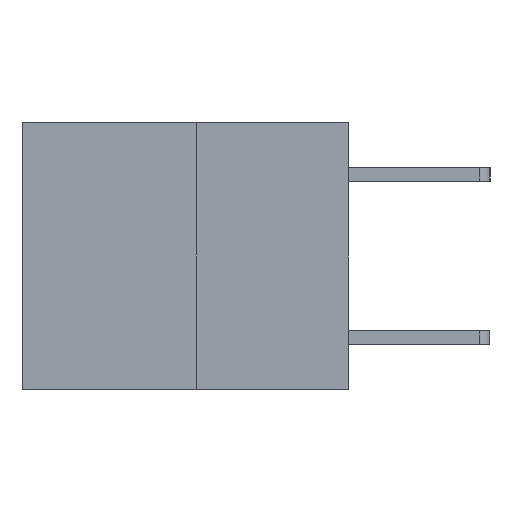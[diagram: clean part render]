
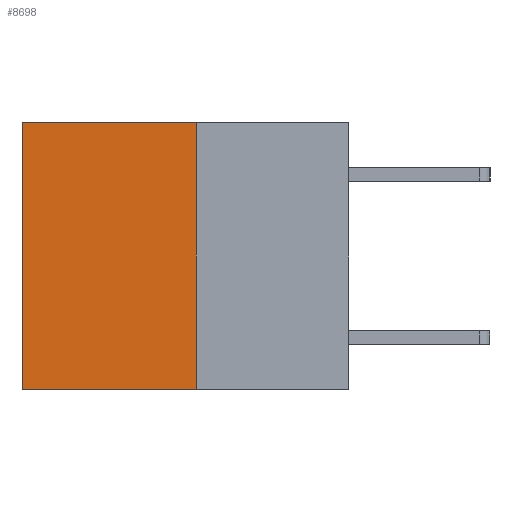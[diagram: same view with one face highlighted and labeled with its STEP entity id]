
A CAD part, left-side view. The second image highlights one B-rep face of the part: STEP entity #8698.
In plain terms, the highlighted planar face has unit normal (-1, 0, 0).
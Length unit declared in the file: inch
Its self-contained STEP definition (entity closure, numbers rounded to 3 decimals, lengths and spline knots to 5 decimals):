
#614 = CARTESIAN_POINT ( 'NONE',  ( 0.3165, 0.28, 0. ) ) ;
#902 = CARTESIAN_POINT ( 'NONE',  ( 0.3165, 0.6, -0.49 ) ) ;
#940 = LINE ( 'NONE', #8660, #9316 ) ;
#1501 = LINE ( 'NONE', #3664, #8991 ) ;
#1710 = VERTEX_POINT ( 'NONE', #614 ) ;
#2042 = DIRECTION ( 'NONE',  ( 0., 1., 0. ) ) ;
#2118 = VERTEX_POINT ( 'NONE', #8180 ) ;
#2866 = EDGE_CURVE ( 'NONE', #1710, #3862, #1501, .T. ) ;
#3375 = DIRECTION ( 'NONE',  ( 0., 0., -1. ) ) ;
#3664 = CARTESIAN_POINT ( 'NONE',  ( 0.3165, 0.28, 0. ) ) ;
#3818 = EDGE_CURVE ( 'NONE', #2118, #5429, #7157, .T. ) ;
#3862 = VERTEX_POINT ( 'NONE', #6712 ) ;
#3995 = DIRECTION ( 'NONE',  ( 0., 0., -1. ) ) ;
#4479 = VECTOR ( 'NONE', #9970, 39.37008 ) ;
#4539 = LINE ( 'NONE', #8281, #8890 ) ;
#5429 = VERTEX_POINT ( 'NONE', #902 ) ;
#6252 = FACE_OUTER_BOUND ( 'NONE', #7639, .T. ) ;
#6377 = CARTESIAN_POINT ( 'NONE',  ( 0.3165, 0.28, -0.49 ) ) ;
#6712 = CARTESIAN_POINT ( 'NONE',  ( 0.3165, 0.6, 0. ) ) ;
#6842 = ORIENTED_EDGE ( 'NONE', *, *, #3818, .F. ) ;
#7156 = CARTESIAN_POINT ( 'NONE',  ( 0.3165, 0.28, -0.49 ) ) ;
#7157 = LINE ( 'NONE', #7156, #4479 ) ;
#7330 = PLANE ( 'NONE',  #8724 ) ;
#7483 = EDGE_CURVE ( 'NONE', #3862, #5429, #4539, .T. ) ;
#7639 = EDGE_LOOP ( 'NONE', ( #8828, #6842, #7789, #8587 ) ) ;
#7755 = DIRECTION ( 'NONE',  ( 0., 0., -1. ) ) ;
#7789 = ORIENTED_EDGE ( 'NONE', *, *, #9198, .F. ) ;
#8180 = CARTESIAN_POINT ( 'NONE',  ( 0.3165, 0.28, -0.49 ) ) ;
#8281 = CARTESIAN_POINT ( 'NONE',  ( 0.3165, 0.6, -0.49 ) ) ;
#8587 = ORIENTED_EDGE ( 'NONE', *, *, #2866, .T. ) ;
#8660 = CARTESIAN_POINT ( 'NONE',  ( 0.3165, 0.28, -0.49 ) ) ;
#8698 = ADVANCED_FACE ( 'NONE', ( #6252 ), #7330, .F. ) ;
#8724 = AXIS2_PLACEMENT_3D ( 'NONE', #6377, #8884, #3995 ) ;
#8828 = ORIENTED_EDGE ( 'NONE', *, *, #7483, .T. ) ;
#8884 = DIRECTION ( 'NONE',  ( 1., 0., 0. ) ) ;
#8890 = VECTOR ( 'NONE', #3375, 39.37008 ) ;
#8991 = VECTOR ( 'NONE', #2042, 39.37008 ) ;
#9198 = EDGE_CURVE ( 'NONE', #1710, #2118, #940, .T. ) ;
#9316 = VECTOR ( 'NONE', #7755, 39.37008 ) ;
#9970 = DIRECTION ( 'NONE',  ( 0., 1., 0. ) ) ;
